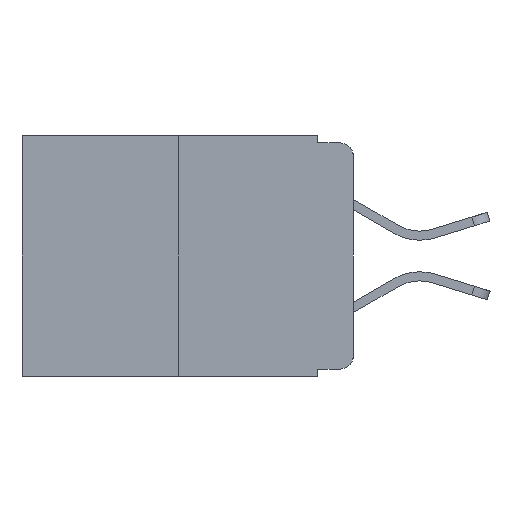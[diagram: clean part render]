
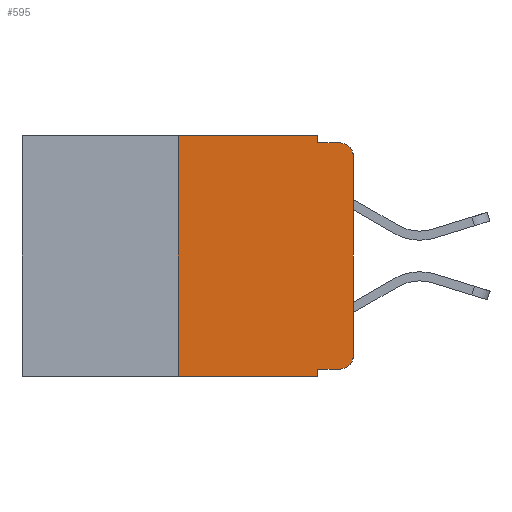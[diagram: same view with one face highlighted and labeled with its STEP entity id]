
A CAD part, left-side view. The second image highlights one B-rep face of the part: STEP entity #595.
In plain terms, the highlighted planar face has unit normal (-1, 0, 0).
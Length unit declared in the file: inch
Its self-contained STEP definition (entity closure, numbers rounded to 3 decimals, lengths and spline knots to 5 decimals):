
#87 = EDGE_CURVE ( 'NONE', #16248, #8477, #19339, .T. ) ;
#144 = LINE ( 'NONE', #12020, #5855 ) ;
#374 = LINE ( 'NONE', #6764, #17814 ) ;
#392 = DIRECTION ( 'NONE',  ( 0., 0., -1. ) ) ;
#525 = VECTOR ( 'NONE', #392, 39.37008 ) ;
#595 = ADVANCED_FACE ( 'NONE', ( #19646 ), #6188, .F. ) ;
#648 = LINE ( 'NONE', #5927, #2905 ) ;
#879 = VECTOR ( 'NONE', #19733, 39.37008 ) ;
#1697 = CARTESIAN_POINT ( 'NONE',  ( 0., 0.02, -0.03 ) ) ;
#1897 = AXIS2_PLACEMENT_3D ( 'NONE', #6406, #9300, #21544 ) ;
#1898 = VERTEX_POINT ( 'NONE', #4208 ) ;
#2098 = CARTESIAN_POINT ( 'NONE',  ( 0., 0., 0. ) ) ;
#2576 = CARTESIAN_POINT ( 'NONE',  ( 0., 0.051, -0.01 ) ) ;
#2899 = CARTESIAN_POINT ( 'NONE',  ( 0., 0., -0.03 ) ) ;
#2905 = VECTOR ( 'NONE', #3926, 39.37008 ) ;
#3926 = DIRECTION ( 'NONE',  ( 0., 0., -1. ) ) ;
#3929 = VERTEX_POINT ( 'NONE', #20201 ) ;
#4159 = EDGE_CURVE ( 'NONE', #8477, #10030, #6057, .T. ) ;
#4208 = CARTESIAN_POINT ( 'NONE',  ( 0., 0.02, -0.333 ) ) ;
#4244 = EDGE_CURVE ( 'NONE', #3929, #8198, #17626, .T. ) ;
#4529 = AXIS2_PLACEMENT_3D ( 'NONE', #20604, #12074, #18925 ) ;
#4720 = DIRECTION ( 'NONE',  ( 0., -1., 0. ) ) ;
#4797 = ORIENTED_EDGE ( 'NONE', *, *, #7411, .F. ) ;
#5855 = VECTOR ( 'NONE', #12358, 39.37008 ) ;
#5927 = CARTESIAN_POINT ( 'NONE',  ( 0., 0.051, 0. ) ) ;
#6057 = LINE ( 'NONE', #2576, #879 ) ;
#6188 = PLANE ( 'NONE',  #1897 ) ;
#6406 = CARTESIAN_POINT ( 'NONE',  ( 0., 0.473, 0. ) ) ;
#6644 = ORIENTED_EDGE ( 'NONE', *, *, #87, .F. ) ;
#6742 = VERTEX_POINT ( 'NONE', #8686 ) ;
#6764 = CARTESIAN_POINT ( 'NONE',  ( 0., 0.051, -0.333 ) ) ;
#6931 = CARTESIAN_POINT ( 'NONE',  ( 0., 0.02, -0.01 ) ) ;
#7207 = VECTOR ( 'NONE', #15790, 39.37008 ) ;
#7411 = EDGE_CURVE ( 'NONE', #3929, #6742, #9735, .T. ) ;
#7557 = CARTESIAN_POINT ( 'NONE',  ( 0., 0.051, -0.333 ) ) ;
#7712 = CARTESIAN_POINT ( 'NONE',  ( 0., 0., -0.313 ) ) ;
#7821 = ORIENTED_EDGE ( 'NONE', *, *, #14577, .T. ) ;
#8056 = DIRECTION ( 'NONE',  ( 0., 0., 1. ) ) ;
#8175 = EDGE_CURVE ( 'NONE', #1898, #15609, #9491, .T. ) ;
#8198 = VERTEX_POINT ( 'NONE', #12635 ) ;
#8477 = VERTEX_POINT ( 'NONE', #20691 ) ;
#8686 = CARTESIAN_POINT ( 'NONE',  ( 0., 0.25, 0. ) ) ;
#8736 = DIRECTION ( 'NONE',  ( -1., 0., 0. ) ) ;
#9018 = ORIENTED_EDGE ( 'NONE', *, *, #9168, .T. ) ;
#9066 = CARTESIAN_POINT ( 'NONE',  ( 0., 0.473, -0.343 ) ) ;
#9168 = EDGE_CURVE ( 'NONE', #21051, #1898, #374, .T. ) ;
#9300 = DIRECTION ( 'NONE',  ( 1., 0., 0. ) ) ;
#9491 = CIRCLE ( 'NONE', #4529, 0.02 ) ;
#9507 = CIRCLE ( 'NONE', #19236, 0.02 ) ;
#9735 = LINE ( 'NONE', #21539, #14237 ) ;
#10030 = VERTEX_POINT ( 'NONE', #6931 ) ;
#10450 = CARTESIAN_POINT ( 'NONE',  ( 0., 0.051, 0. ) ) ;
#10771 = DIRECTION ( 'NONE',  ( 0., -1., 0. ) ) ;
#10798 = CARTESIAN_POINT ( 'NONE',  ( 0., 0.051, 0. ) ) ;
#11414 = EDGE_LOOP ( 'NONE', ( #7821, #20056, #12944, #6644, #17762, #4797, #18339, #12598, #9018, #20592 ) ) ;
#12020 = CARTESIAN_POINT ( 'NONE',  ( 0., 0.473, 0. ) ) ;
#12045 = VECTOR ( 'NONE', #4720, 39.37008 ) ;
#12074 = DIRECTION ( 'NONE',  ( -1., 0., 0. ) ) ;
#12358 = DIRECTION ( 'NONE',  ( 0., -1., 0. ) ) ;
#12598 = ORIENTED_EDGE ( 'NONE', *, *, #12727, .F. ) ;
#12635 = CARTESIAN_POINT ( 'NONE',  ( 0., 0.051, -0.343 ) ) ;
#12727 = EDGE_CURVE ( 'NONE', #21051, #8198, #648, .T. ) ;
#12944 = ORIENTED_EDGE ( 'NONE', *, *, #4159, .F. ) ;
#14237 = VECTOR ( 'NONE', #8056, 39.37008 ) ;
#14577 = EDGE_CURVE ( 'NONE', #15609, #15500, #17467, .T. ) ;
#15268 = DIRECTION ( 'NONE',  ( 0., 0., -1. ) ) ;
#15500 = VERTEX_POINT ( 'NONE', #2899 ) ;
#15609 = VERTEX_POINT ( 'NONE', #7712 ) ;
#15790 = DIRECTION ( 'NONE',  ( 0., 0., 1. ) ) ;
#16248 = VERTEX_POINT ( 'NONE', #10798 ) ;
#16646 = EDGE_CURVE ( 'NONE', #6742, #16248, #144, .T. ) ;
#17467 = LINE ( 'NONE', #2098, #7207 ) ;
#17626 = LINE ( 'NONE', #9066, #12045 ) ;
#17762 = ORIENTED_EDGE ( 'NONE', *, *, #16646, .F. ) ;
#17814 = VECTOR ( 'NONE', #10771, 39.37008 ) ;
#18339 = ORIENTED_EDGE ( 'NONE', *, *, #4244, .T. ) ;
#18925 = DIRECTION ( 'NONE',  ( 0., 0., -1. ) ) ;
#19236 = AXIS2_PLACEMENT_3D ( 'NONE', #1697, #8736, #15268 ) ;
#19339 = LINE ( 'NONE', #10450, #525 ) ;
#19646 = FACE_OUTER_BOUND ( 'NONE', #11414, .T. ) ;
#19733 = DIRECTION ( 'NONE',  ( 0., -1., 0. ) ) ;
#20056 = ORIENTED_EDGE ( 'NONE', *, *, #21915, .T. ) ;
#20201 = CARTESIAN_POINT ( 'NONE',  ( 0., 0.25, -0.343 ) ) ;
#20592 = ORIENTED_EDGE ( 'NONE', *, *, #8175, .T. ) ;
#20604 = CARTESIAN_POINT ( 'NONE',  ( 0., 0.02, -0.313 ) ) ;
#20691 = CARTESIAN_POINT ( 'NONE',  ( 0., 0.051, -0.01 ) ) ;
#21051 = VERTEX_POINT ( 'NONE', #7557 ) ;
#21539 = CARTESIAN_POINT ( 'NONE',  ( 0., 0.25, 0. ) ) ;
#21544 = DIRECTION ( 'NONE',  ( 0., 0., -1. ) ) ;
#21915 = EDGE_CURVE ( 'NONE', #15500, #10030, #9507, .T. ) ;
